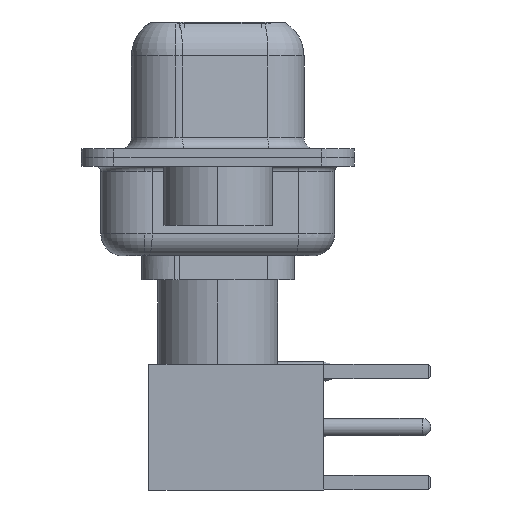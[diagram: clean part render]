
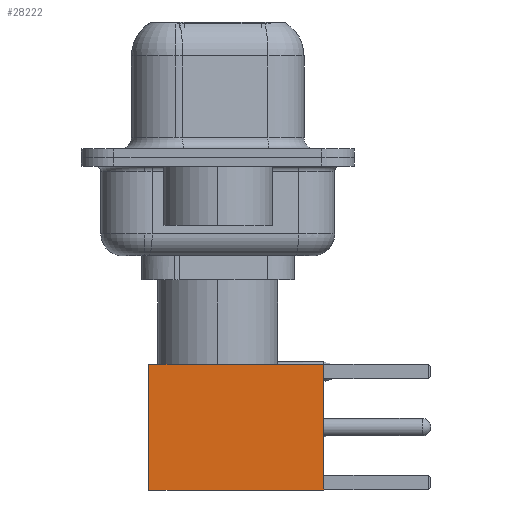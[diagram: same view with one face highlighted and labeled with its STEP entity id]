
A CAD part, left-side view. The second image highlights one B-rep face of the part: STEP entity #28222.
In plain terms, the highlighted face is planar.
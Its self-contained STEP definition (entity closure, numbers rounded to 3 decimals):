
#930 = EDGE_CURVE ( 'NONE', #974, #16937, #25951, .T. ) ;
#974 = VERTEX_POINT ( 'NONE', #20222 ) ;
#1048 = DIRECTION ( 'NONE',  ( 0., 0., 1. ) ) ;
#2518 = LINE ( 'NONE', #11259, #16643 ) ;
#2615 = DIRECTION ( 'NONE',  ( 0., 0., -1. ) ) ;
#3196 = DIRECTION ( 'NONE',  ( 0., 1., 0. ) ) ;
#4355 = AXIS2_PLACEMENT_3D ( 'NONE', #7051, #3196, #1048 ) ;
#4750 = CARTESIAN_POINT ( 'NONE',  ( 2.875, 2.875, 0. ) ) ;
#5710 = DIRECTION ( 'NONE',  ( -1., 0., 0. ) ) ;
#5843 = CARTESIAN_POINT ( 'NONE',  ( 0., 2.875, 8. ) ) ;
#6720 = EDGE_CURVE ( 'NONE', #8888, #16937, #2518, .T. ) ;
#7051 = CARTESIAN_POINT ( 'NONE',  ( 2.875, 2.875, 0. ) ) ;
#7876 = CARTESIAN_POINT ( 'NONE',  ( -2.875, 2.875, 0. ) ) ;
#8803 = CARTESIAN_POINT ( 'NONE',  ( 2.875, 2.875, 8. ) ) ;
#8888 = VERTEX_POINT ( 'NONE', #16614 ) ;
#9386 = ORIENTED_EDGE ( 'NONE', *, *, #24432, .F. ) ;
#11259 = CARTESIAN_POINT ( 'NONE',  ( -2.875, 2.875, 0. ) ) ;
#11829 = VERTEX_POINT ( 'NONE', #8803 ) ;
#11992 = VECTOR ( 'NONE', #5710, 1000. ) ;
#12946 = CARTESIAN_POINT ( 'NONE',  ( 0., 2.875, 0. ) ) ;
#14104 = VECTOR ( 'NONE', #2615, 1000. ) ;
#14792 = DIRECTION ( 'NONE',  ( -1., 0., 0. ) ) ;
#14839 = ORIENTED_EDGE ( 'NONE', *, *, #19536, .T. ) ;
#15066 = EDGE_LOOP ( 'NONE', ( #14839, #17995, #20533, #9386 ) ) ;
#16614 = CARTESIAN_POINT ( 'NONE',  ( -2.875, 2.875, 8. ) ) ;
#16643 = VECTOR ( 'NONE', #20009, 1000. ) ;
#16937 = VERTEX_POINT ( 'NONE', #7876 ) ;
#17995 = ORIENTED_EDGE ( 'NONE', *, *, #930, .T. ) ;
#19536 = EDGE_CURVE ( 'NONE', #11829, #974, #26792, .T. ) ;
#20009 = DIRECTION ( 'NONE',  ( 0., 0., -1. ) ) ;
#20222 = CARTESIAN_POINT ( 'NONE',  ( 2.875, 2.875, 0. ) ) ;
#20533 = ORIENTED_EDGE ( 'NONE', *, *, #6720, .F. ) ;
#20669 = PLANE ( 'NONE',  #4355 ) ;
#22810 = FACE_OUTER_BOUND ( 'NONE', #15066, .T. ) ;
#24432 = EDGE_CURVE ( 'NONE', #11829, #8888, #27461, .T. ) ;
#25324 = VECTOR ( 'NONE', #14792, 1000. ) ;
#25951 = LINE ( 'NONE', #12946, #25324 ) ;
#26792 = LINE ( 'NONE', #4750, #14104 ) ;
#27461 = LINE ( 'NONE', #5843, #11992 ) ;
#28222 = ADVANCED_FACE ( 'NONE', ( #22810 ), #20669, .T. ) ;
